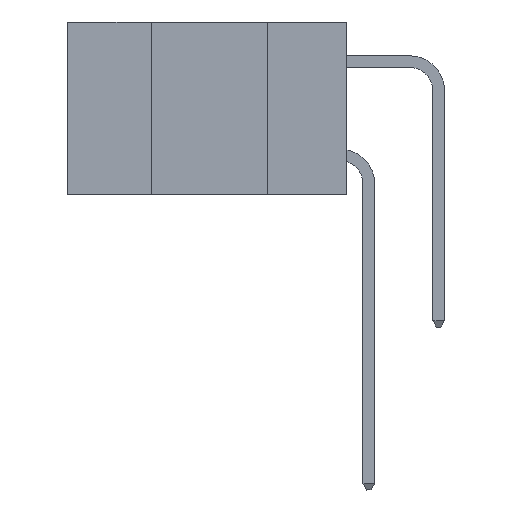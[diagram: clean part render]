
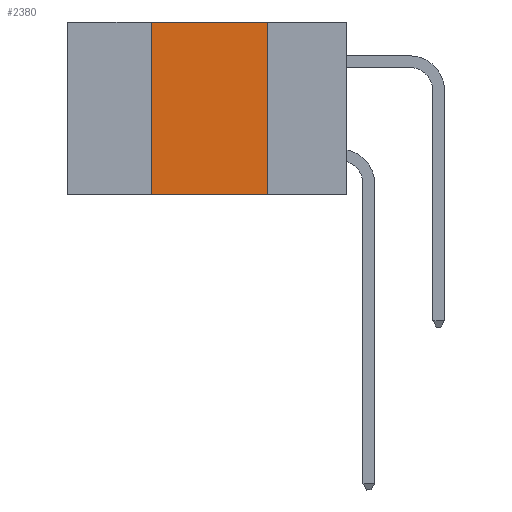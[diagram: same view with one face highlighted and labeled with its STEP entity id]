
A CAD part, left-side view. The second image highlights one B-rep face of the part: STEP entity #2380.
In plain terms, the highlighted planar face has unit normal (-1, 0, 0).
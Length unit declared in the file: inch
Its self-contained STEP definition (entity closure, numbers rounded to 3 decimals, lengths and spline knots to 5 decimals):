
#1776 = EDGE_CURVE ( 'NONE', #13317, #28902, #25324, .T. ) ;
#2272 = CARTESIAN_POINT ( 'NONE',  ( 0., 0.6, -0.37 ) ) ;
#2380 = ADVANCED_FACE ( 'NONE', ( #19190 ), #2381, .F. ) ;
#2381 = PLANE ( 'NONE',  #21051 ) ;
#4664 = LINE ( 'NONE', #12510, #24396 ) ;
#4890 = DIRECTION ( 'NONE',  ( 0., 0., -1. ) ) ;
#5558 = DIRECTION ( 'NONE',  ( 0., 0., -1. ) ) ;
#6002 = EDGE_LOOP ( 'NONE', ( #32419, #20207, #16727, #23446 ) ) ;
#9890 = DIRECTION ( 'NONE',  ( 0., -1., 0. ) ) ;
#9989 = DIRECTION ( 'NONE',  ( 1., 0., 0. ) ) ;
#11653 = VERTEX_POINT ( 'NONE', #21253 ) ;
#12510 = CARTESIAN_POINT ( 'NONE',  ( 0., 0.6, 0. ) ) ;
#12873 = CARTESIAN_POINT ( 'NONE',  ( 0., 0.42, 0. ) ) ;
#13317 = VERTEX_POINT ( 'NONE', #29446 ) ;
#13557 = VECTOR ( 'NONE', #4890, 39.37008 ) ;
#13820 = LINE ( 'NONE', #12873, #19072 ) ;
#15273 = CARTESIAN_POINT ( 'NONE',  ( 0., 0.17, 0. ) ) ;
#16727 = ORIENTED_EDGE ( 'NONE', *, *, #21730, .F. ) ;
#18312 = DIRECTION ( 'NONE',  ( 0., 0., 1. ) ) ;
#19072 = VECTOR ( 'NONE', #18312, 39.37008 ) ;
#19190 = FACE_OUTER_BOUND ( 'NONE', #6002, .T. ) ;
#19472 = VERTEX_POINT ( 'NONE', #24157 ) ;
#19573 = EDGE_CURVE ( 'NONE', #11653, #13317, #4664, .T. ) ;
#20030 = LINE ( 'NONE', #2272, #24900 ) ;
#20207 = ORIENTED_EDGE ( 'NONE', *, *, #19573, .F. ) ;
#21051 = AXIS2_PLACEMENT_3D ( 'NONE', #25439, #9989, #5558 ) ;
#21253 = CARTESIAN_POINT ( 'NONE',  ( 0., 0.42, 0. ) ) ;
#21730 = EDGE_CURVE ( 'NONE', #19472, #11653, #13820, .T. ) ;
#23446 = ORIENTED_EDGE ( 'NONE', *, *, #24950, .T. ) ;
#24157 = CARTESIAN_POINT ( 'NONE',  ( 0., 0.42, -0.37 ) ) ;
#24396 = VECTOR ( 'NONE', #33101, 39.37008 ) ;
#24900 = VECTOR ( 'NONE', #9890, 39.37008 ) ;
#24950 = EDGE_CURVE ( 'NONE', #19472, #28902, #20030, .T. ) ;
#25324 = LINE ( 'NONE', #15273, #13557 ) ;
#25439 = CARTESIAN_POINT ( 'NONE',  ( 0., 0.6, 0. ) ) ;
#25832 = CARTESIAN_POINT ( 'NONE',  ( 0., 0.17, -0.37 ) ) ;
#28902 = VERTEX_POINT ( 'NONE', #25832 ) ;
#29446 = CARTESIAN_POINT ( 'NONE',  ( 0., 0.17, 0. ) ) ;
#32419 = ORIENTED_EDGE ( 'NONE', *, *, #1776, .F. ) ;
#33101 = DIRECTION ( 'NONE',  ( 0., -1., 0. ) ) ;
